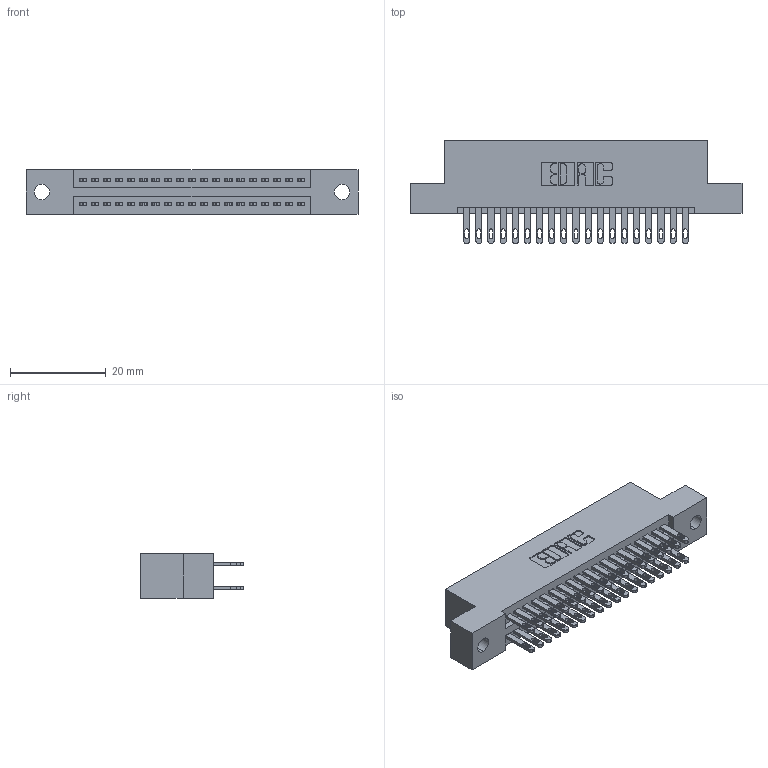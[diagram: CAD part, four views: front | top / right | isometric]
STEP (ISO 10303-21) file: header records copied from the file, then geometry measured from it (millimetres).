
FILE_DESCRIPTION (( 'STEP AP203' ), '1' );
FILE_NAME ('895-038-500-202.STEP', '2020-09-26T00:52:30', ( '' ), ( '' ), 'SwSTEP 2.0', 'SolidWorks 2020', '' );
FILE_SCHEMA (( 'CONFIG_CONTROL_DESIGN' ));
Length unit declared in the file: inch
Products named in the file (3): 845 Part_Flush Mounting Lugs - 0.128 Dia; 345-292-001_345-293-100; 895-038-500-202
Assembly tree (39 placements, depth 2):
  895-038-500-202
    845 Part_Flush Mounting Lugs - 0.128 Dia
    345-292-001_345-293-100  x38
Bounding box: 69.47 x 21.51 x 9.4 mm (x, y, z)
Volume: 6614.2 mm3; surface area: 9446.3 mm2
Topology: 39 solids, 39 shells, 1874 faces, 5699 edges, 3798 vertices
Faces by surface type: plane 1106, cylinder 768
Entity records: 17937 total; most frequent: CARTESIAN_POINT 3028, ORIENTED_EDGE 2962, DIRECTION 2701, EDGE_CURVE 1481, LINE 1269, VECTOR 1269, VERTEX_POINT 986, AXIS2_PLACEMENT_3D 716
